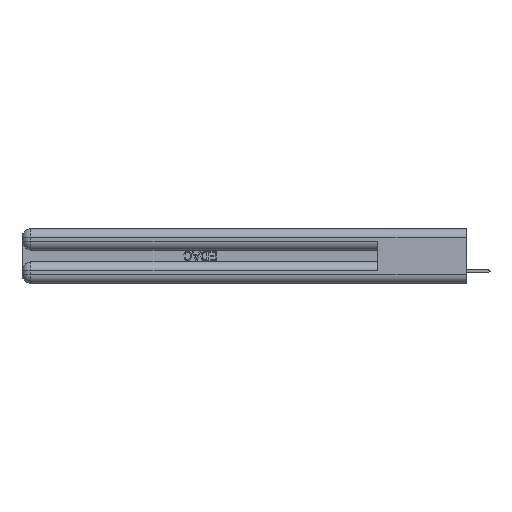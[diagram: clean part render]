
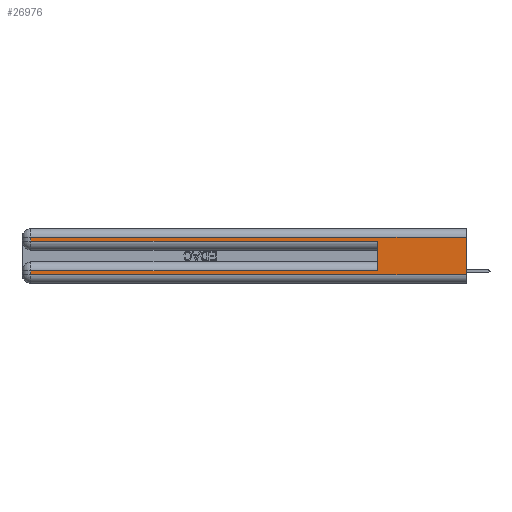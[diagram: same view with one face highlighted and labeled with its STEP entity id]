
A CAD part, left-side view. The second image highlights one B-rep face of the part: STEP entity #26976.
In plain terms, the highlighted planar face has unit normal (-1, 0, 0).
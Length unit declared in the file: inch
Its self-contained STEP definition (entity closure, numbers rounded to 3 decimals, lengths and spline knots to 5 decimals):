
#508 = EDGE_CURVE ( 'NONE', #10388, #13631, #22288, .T. ) ;
#1137 = EDGE_CURVE ( 'NONE', #13444, #10181, #1956, .T. ) ;
#1540 = EDGE_LOOP ( 'NONE', ( #19906, #29028, #7162, #22168, #18227, #14388, #4804, #36612 ) ) ;
#1956 = LINE ( 'NONE', #32715, #15486 ) ;
#3253 = VERTEX_POINT ( 'NONE', #33306 ) ;
#3718 = CARTESIAN_POINT ( 'NONE',  ( 0., 2.94, 0.37 ) ) ;
#4586 = DIRECTION ( 'NONE',  ( 0., 1., 0. ) ) ;
#4804 = ORIENTED_EDGE ( 'NONE', *, *, #30351, .T. ) ;
#4894 = CARTESIAN_POINT ( 'NONE',  ( 0., 0.6, 0.145 ) ) ;
#5486 = LINE ( 'NONE', #3718, #8106 ) ;
#6618 = VECTOR ( 'NONE', #29789, 39.37008 ) ;
#7162 = ORIENTED_EDGE ( 'NONE', *, *, #20480, .T. ) ;
#8045 = AXIS2_PLACEMENT_3D ( 'NONE', #33427, #34571, #24665 ) ;
#8106 = VECTOR ( 'NONE', #20521, 39.37008 ) ;
#8903 = LINE ( 'NONE', #20646, #17094 ) ;
#10181 = VERTEX_POINT ( 'NONE', #27952 ) ;
#10388 = VERTEX_POINT ( 'NONE', #16898 ) ;
#11937 = VECTOR ( 'NONE', #14396, 39.37008 ) ;
#13444 = VERTEX_POINT ( 'NONE', #14885 ) ;
#13631 = VERTEX_POINT ( 'NONE', #38647 ) ;
#14388 = ORIENTED_EDGE ( 'NONE', *, *, #508, .T. ) ;
#14396 = DIRECTION ( 'NONE',  ( 0., 1., 0. ) ) ;
#14885 = CARTESIAN_POINT ( 'NONE',  ( 0., 2.94, 0.285 ) ) ;
#15486 = VECTOR ( 'NONE', #35182, 39.37008 ) ;
#16701 = VERTEX_POINT ( 'NONE', #17013 ) ;
#16736 = CARTESIAN_POINT ( 'NONE',  ( 0., 0., 0.085 ) ) ;
#16898 = CARTESIAN_POINT ( 'NONE',  ( 0., 0.6, 0.085 ) ) ;
#17013 = CARTESIAN_POINT ( 'NONE',  ( 0., 2.94, 0.06 ) ) ;
#17094 = VECTOR ( 'NONE', #4586, 39.37008 ) ;
#18140 = VERTEX_POINT ( 'NONE', #29421 ) ;
#18227 = ORIENTED_EDGE ( 'NONE', *, *, #20898, .F. ) ;
#18483 = VERTEX_POINT ( 'NONE', #34503 ) ;
#19906 = ORIENTED_EDGE ( 'NONE', *, *, #22297, .F. ) ;
#19907 = FACE_OUTER_BOUND ( 'NONE', #1540, .T. ) ;
#20480 = EDGE_CURVE ( 'NONE', #3253, #13444, #27455, .T. ) ;
#20521 = DIRECTION ( 'NONE',  ( 0., 0., -1. ) ) ;
#20646 = CARTESIAN_POINT ( 'NONE',  ( 0., 0., 0.31 ) ) ;
#20898 = EDGE_CURVE ( 'NONE', #10388, #10181, #22830, .T. ) ;
#22168 = ORIENTED_EDGE ( 'NONE', *, *, #1137, .T. ) ;
#22288 = LINE ( 'NONE', #16736, #11937 ) ;
#22297 = EDGE_CURVE ( 'NONE', #18483, #18140, #38328, .T. ) ;
#22830 = LINE ( 'NONE', #4894, #39961 ) ;
#24665 = DIRECTION ( 'NONE',  ( 0., 0., -1. ) ) ;
#25662 = CARTESIAN_POINT ( 'NONE',  ( 0., 2.94, 0.37 ) ) ;
#25769 = LINE ( 'NONE', #26310, #6618 ) ;
#25969 = DIRECTION ( 'NONE',  ( 0., 0., -1. ) ) ;
#26310 = CARTESIAN_POINT ( 'NONE',  ( 0., 0., 0.06 ) ) ;
#26976 = ADVANCED_FACE ( 'NONE', ( #19907 ), #30093, .F. ) ;
#27455 = LINE ( 'NONE', #25662, #39502 ) ;
#27540 = DIRECTION ( 'NONE',  ( 0., 0., -1. ) ) ;
#27952 = CARTESIAN_POINT ( 'NONE',  ( 0., 0.6, 0.285 ) ) ;
#29028 = ORIENTED_EDGE ( 'NONE', *, *, #39650, .T. ) ;
#29421 = CARTESIAN_POINT ( 'NONE',  ( 0., 0., 0.06 ) ) ;
#29625 = EDGE_CURVE ( 'NONE', #16701, #18140, #25769, .T. ) ;
#29789 = DIRECTION ( 'NONE',  ( 0., -1., 0. ) ) ;
#30093 = PLANE ( 'NONE',  #8045 ) ;
#30351 = EDGE_CURVE ( 'NONE', #13631, #16701, #5486, .T. ) ;
#30528 = VECTOR ( 'NONE', #27540, 39.37008 ) ;
#32715 = CARTESIAN_POINT ( 'NONE',  ( 0., 0., 0.285 ) ) ;
#33306 = CARTESIAN_POINT ( 'NONE',  ( 0., 2.94, 0.31 ) ) ;
#33427 = CARTESIAN_POINT ( 'NONE',  ( 0., 0., 0.37 ) ) ;
#34241 = CARTESIAN_POINT ( 'NONE',  ( 0., 0., 0.37 ) ) ;
#34503 = CARTESIAN_POINT ( 'NONE',  ( 0., 0., 0.31 ) ) ;
#34571 = DIRECTION ( 'NONE',  ( 1., 0., 0. ) ) ;
#35057 = DIRECTION ( 'NONE',  ( 0., 0., 1. ) ) ;
#35182 = DIRECTION ( 'NONE',  ( 0., -1., 0. ) ) ;
#36612 = ORIENTED_EDGE ( 'NONE', *, *, #29625, .T. ) ;
#38328 = LINE ( 'NONE', #34241, #30528 ) ;
#38647 = CARTESIAN_POINT ( 'NONE',  ( 0., 2.94, 0.085 ) ) ;
#39502 = VECTOR ( 'NONE', #25969, 39.37008 ) ;
#39650 = EDGE_CURVE ( 'NONE', #18483, #3253, #8903, .T. ) ;
#39961 = VECTOR ( 'NONE', #35057, 39.37008 ) ;
